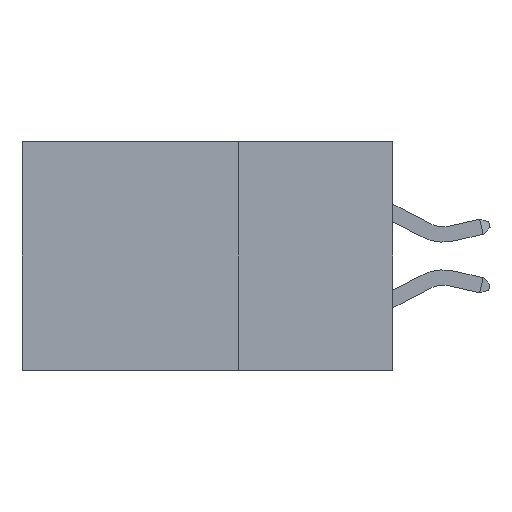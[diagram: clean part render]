
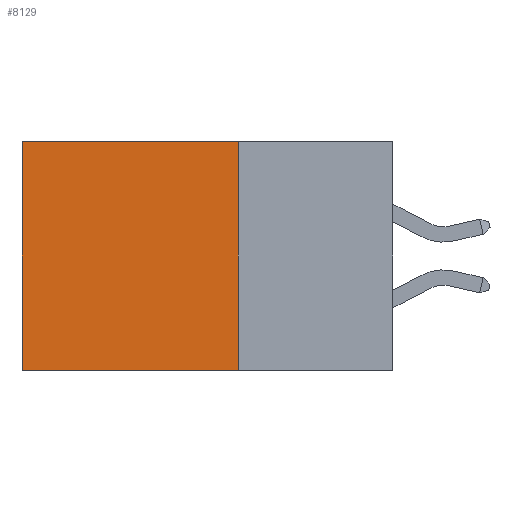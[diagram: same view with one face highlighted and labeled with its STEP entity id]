
A CAD part, left-side view. The second image highlights one B-rep face of the part: STEP entity #8129.
In plain terms, the highlighted planar face has unit normal (-1, 0, 0).
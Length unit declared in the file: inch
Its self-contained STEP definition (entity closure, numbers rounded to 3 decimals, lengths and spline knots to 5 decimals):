
#220 = LINE ( 'NONE', #3163, #6464 ) ;
#640 = DIRECTION ( 'NONE',  ( 0., 1., 0. ) ) ;
#918 = VERTEX_POINT ( 'NONE', #2877 ) ;
#1114 = AXIS2_PLACEMENT_3D ( 'NONE', #11874, #3386, #10875 ) ;
#1240 = CARTESIAN_POINT ( 'NONE',  ( 0.2875, 0.25, 0. ) ) ;
#1814 = ORIENTED_EDGE ( 'NONE', *, *, #10236, .F. ) ;
#1823 = VERTEX_POINT ( 'NONE', #9989 ) ;
#2003 = VERTEX_POINT ( 'NONE', #3489 ) ;
#2325 = CARTESIAN_POINT ( 'NONE',  ( 0.2875, 0.6, 0. ) ) ;
#2844 = EDGE_LOOP ( 'NONE', ( #7949, #1814, #3221, #4508 ) ) ;
#2877 = CARTESIAN_POINT ( 'NONE',  ( 0.2875, 0.6, -0.37 ) ) ;
#3163 = CARTESIAN_POINT ( 'NONE',  ( 0.2875, 0.25, -0.37 ) ) ;
#3221 = ORIENTED_EDGE ( 'NONE', *, *, #5373, .F. ) ;
#3386 = DIRECTION ( 'NONE',  ( 1., 0., 0. ) ) ;
#3489 = CARTESIAN_POINT ( 'NONE',  ( 0.2875, 0.25, 0. ) ) ;
#3917 = EDGE_CURVE ( 'NONE', #2003, #1823, #11967, .T. ) ;
#4088 = DIRECTION ( 'NONE',  ( 0., 0., -1. ) ) ;
#4319 = VECTOR ( 'NONE', #4088, 39.37008 ) ;
#4508 = ORIENTED_EDGE ( 'NONE', *, *, #3917, .T. ) ;
#4986 = DIRECTION ( 'NONE',  ( 0., 0., -1. ) ) ;
#5134 = DIRECTION ( 'NONE',  ( 0., 1., 0. ) ) ;
#5373 = EDGE_CURVE ( 'NONE', #2003, #6777, #9642, .T. ) ;
#5414 = CARTESIAN_POINT ( 'NONE',  ( 0.2875, 0.25, -0.37 ) ) ;
#6328 = FACE_OUTER_BOUND ( 'NONE', #2844, .T. ) ;
#6464 = VECTOR ( 'NONE', #5134, 39.37008 ) ;
#6777 = VERTEX_POINT ( 'NONE', #5414 ) ;
#7949 = ORIENTED_EDGE ( 'NONE', *, *, #9778, .T. ) ;
#8129 = ADVANCED_FACE ( 'NONE', ( #6328 ), #8233, .F. ) ;
#8233 = PLANE ( 'NONE',  #1114 ) ;
#8325 = CARTESIAN_POINT ( 'NONE',  ( 0.2875, 0.25, 0. ) ) ;
#8839 = VECTOR ( 'NONE', #640, 39.37008 ) ;
#9642 = LINE ( 'NONE', #1240, #10144 ) ;
#9778 = EDGE_CURVE ( 'NONE', #1823, #918, #11551, .T. ) ;
#9989 = CARTESIAN_POINT ( 'NONE',  ( 0.2875, 0.6, 0. ) ) ;
#10144 = VECTOR ( 'NONE', #4986, 39.37008 ) ;
#10236 = EDGE_CURVE ( 'NONE', #6777, #918, #220, .T. ) ;
#10875 = DIRECTION ( 'NONE',  ( 0., 0., -1. ) ) ;
#11551 = LINE ( 'NONE', #2325, #4319 ) ;
#11874 = CARTESIAN_POINT ( 'NONE',  ( 0.2875, 0.25, 0. ) ) ;
#11967 = LINE ( 'NONE', #8325, #8839 ) ;
